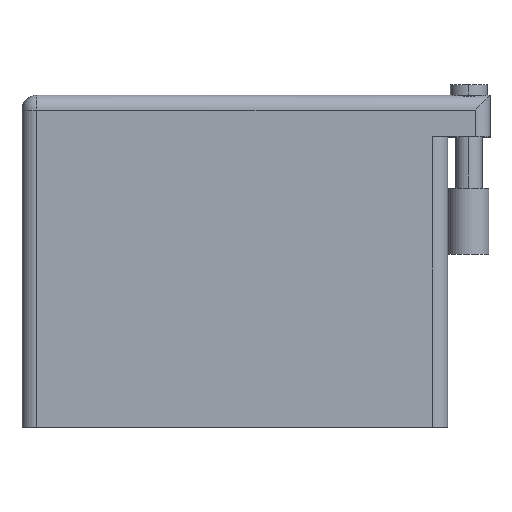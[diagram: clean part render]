
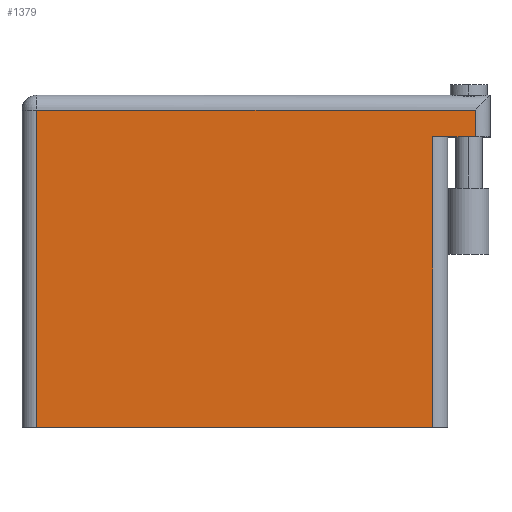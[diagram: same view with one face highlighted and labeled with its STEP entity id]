
A CAD part, top view. The second image highlights one B-rep face of the part: STEP entity #1379.
In plain terms, the highlighted planar face has unit normal (0, 0, 1).
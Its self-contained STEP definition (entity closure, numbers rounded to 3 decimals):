
#127 = CARTESIAN_POINT ( 'NONE',  ( 1.778, 0., 0. ) ) ;
#223 = VERTEX_POINT ( 'NONE', #1983 ) ;
#249 = CARTESIAN_POINT ( 'NONE',  ( 1.778, 37.998, 0. ) ) ;
#280 = VERTEX_POINT ( 'NONE', #768 ) ;
#292 = AXIS2_PLACEMENT_3D ( 'NONE', #1826, #1113, #948 ) ;
#334 = LINE ( 'NONE', #1824, #1066 ) ;
#378 = VECTOR ( 'NONE', #1068, 1000. ) ;
#409 = VERTEX_POINT ( 'NONE', #1385 ) ;
#453 = EDGE_CURVE ( 'NONE', #280, #409, #1559, .T. ) ;
#484 = DIRECTION ( 'NONE',  ( 0., 1., 0. ) ) ;
#534 = ORIENTED_EDGE ( 'NONE', *, *, #582, .T. ) ;
#582 = EDGE_CURVE ( 'NONE', #223, #2034, #1471, .T. ) ;
#649 = CARTESIAN_POINT ( 'NONE',  ( 54.305, 37.998, 0. ) ) ;
#734 = CARTESIAN_POINT ( 'NONE',  ( 56.083, 34.773, 0. ) ) ;
#763 = EDGE_CURVE ( 'NONE', #280, #800, #1317, .T. ) ;
#768 = CARTESIAN_POINT ( 'NONE',  ( 54.305, 34.773, 0. ) ) ;
#800 = VERTEX_POINT ( 'NONE', #649 ) ;
#856 = CARTESIAN_POINT ( 'NONE',  ( 54.305, 39.776, 0. ) ) ;
#948 = DIRECTION ( 'NONE',  ( -1., 0., 0. ) ) ;
#1003 = CARTESIAN_POINT ( 'NONE',  ( 0., 37.998, 0. ) ) ;
#1015 = ORIENTED_EDGE ( 'NONE', *, *, #1781, .T. ) ;
#1050 = CARTESIAN_POINT ( 'NONE',  ( 49.225, 0., 0. ) ) ;
#1066 = VECTOR ( 'NONE', #484, 1000. ) ;
#1068 = DIRECTION ( 'NONE',  ( -1., 0., 0. ) ) ;
#1072 = ORIENTED_EDGE ( 'NONE', *, *, #2195, .T. ) ;
#1087 = VECTOR ( 'NONE', #1670, 1000. ) ;
#1099 = EDGE_CURVE ( 'NONE', #1443, #223, #1452, .T. ) ;
#1113 = DIRECTION ( 'NONE',  ( 0., 0., -1. ) ) ;
#1153 = DIRECTION ( 'NONE',  ( -1., 0., 0. ) ) ;
#1252 = FACE_OUTER_BOUND ( 'NONE', #1966, .T. ) ;
#1317 = LINE ( 'NONE', #856, #1087 ) ;
#1318 = DIRECTION ( 'NONE',  ( 0., -1., 0. ) ) ;
#1379 = ADVANCED_FACE ( 'NONE', ( #1252 ), #1602, .F. ) ;
#1385 = CARTESIAN_POINT ( 'NONE',  ( 49.225, 34.773, 0. ) ) ;
#1443 = VERTEX_POINT ( 'NONE', #249 ) ;
#1452 = LINE ( 'NONE', #127, #1855 ) ;
#1453 = VECTOR ( 'NONE', #2127, 1000. ) ;
#1471 = LINE ( 'NONE', #1961, #1453 ) ;
#1559 = LINE ( 'NONE', #734, #378 ) ;
#1602 = PLANE ( 'NONE',  #292 ) ;
#1670 = DIRECTION ( 'NONE',  ( 0., 1., 0. ) ) ;
#1781 = EDGE_CURVE ( 'NONE', #2034, #409, #334, .T. ) ;
#1823 = ORIENTED_EDGE ( 'NONE', *, *, #1099, .T. ) ;
#1824 = CARTESIAN_POINT ( 'NONE',  ( 49.225, 34.773, 0. ) ) ;
#1826 = CARTESIAN_POINT ( 'NONE',  ( 0., 39.776, 0. ) ) ;
#1832 = ORIENTED_EDGE ( 'NONE', *, *, #763, .T. ) ;
#1855 = VECTOR ( 'NONE', #1318, 1000. ) ;
#1863 = LINE ( 'NONE', #1003, #2138 ) ;
#1961 = CARTESIAN_POINT ( 'NONE',  ( 0., 0., 0. ) ) ;
#1966 = EDGE_LOOP ( 'NONE', ( #534, #1015, #1981, #1832, #1072, #1823 ) ) ;
#1981 = ORIENTED_EDGE ( 'NONE', *, *, #453, .F. ) ;
#1983 = CARTESIAN_POINT ( 'NONE',  ( 1.778, 0., 0. ) ) ;
#2034 = VERTEX_POINT ( 'NONE', #1050 ) ;
#2127 = DIRECTION ( 'NONE',  ( 1., 0., 0. ) ) ;
#2138 = VECTOR ( 'NONE', #1153, 1000. ) ;
#2195 = EDGE_CURVE ( 'NONE', #800, #1443, #1863, .T. ) ;
